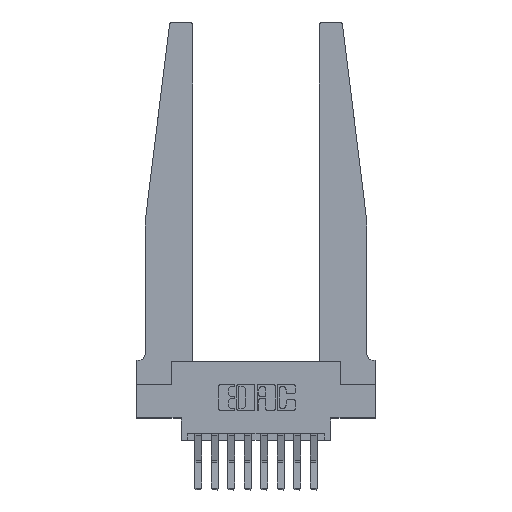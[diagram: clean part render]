
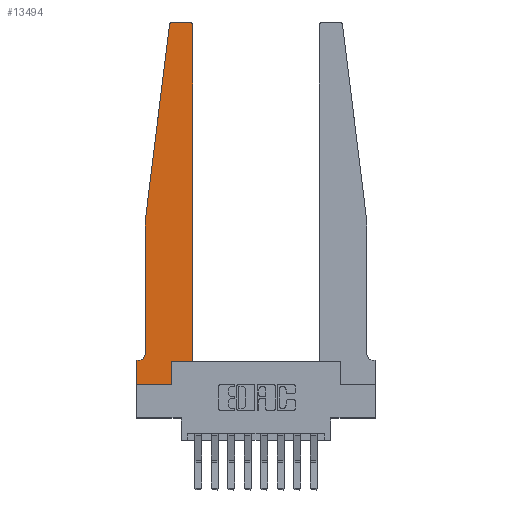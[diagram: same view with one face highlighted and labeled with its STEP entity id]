
A CAD part, top view. The second image highlights one B-rep face of the part: STEP entity #13494.
In plain terms, the highlighted planar face has unit normal (0, 0, 1).
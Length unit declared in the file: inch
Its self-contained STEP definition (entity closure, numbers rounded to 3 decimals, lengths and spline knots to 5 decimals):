
#109 = VECTOR ( 'NONE', #4721, 39.37008 ) ;
#311 = ORIENTED_EDGE ( 'NONE', *, *, #5082, .T. ) ;
#319 = DIRECTION ( 'NONE',  ( 0., 1., 0. ) ) ;
#693 = ORIENTED_EDGE ( 'NONE', *, *, #2034, .T. ) ;
#703 = ORIENTED_EDGE ( 'NONE', *, *, #11220, .T. ) ;
#706 = CARTESIAN_POINT ( 'NONE',  ( 0.27653, 2.72, 0.37 ) ) ;
#908 = AXIS2_PLACEMENT_3D ( 'NONE', #3450, #4506, #8094 ) ;
#1229 = DIRECTION ( 'NONE',  ( 0., -1., 0. ) ) ;
#1250 = EDGE_CURVE ( 'NONE', #2237, #6343, #10101, .T. ) ;
#1474 = LINE ( 'NONE', #10865, #3398 ) ;
#1590 = AXIS2_PLACEMENT_3D ( 'NONE', #5917, #10556, #12864 ) ;
#1916 = VECTOR ( 'NONE', #14478, 39.37008 ) ;
#1954 = VECTOR ( 'NONE', #14543, 39.37008 ) ;
#2034 = EDGE_CURVE ( 'NONE', #4406, #7378, #13529, .T. ) ;
#2237 = VERTEX_POINT ( 'NONE', #14518 ) ;
#2655 = CARTESIAN_POINT ( 'NONE',  ( 0., 0., 0.37 ) ) ;
#2933 = VECTOR ( 'NONE', #10712, 39.37008 ) ;
#3125 = CARTESIAN_POINT ( 'NONE',  ( 0.395, 2.75, 0.37 ) ) ;
#3334 = LINE ( 'NONE', #13623, #9030 ) ;
#3358 = CARTESIAN_POINT ( 'NONE',  ( 0.2605, 0.18, 0.37 ) ) ;
#3398 = VECTOR ( 'NONE', #319, 39.37008 ) ;
#3450 = CARTESIAN_POINT ( 'NONE',  ( 0.395, 2.72, 0.37 ) ) ;
#3584 = EDGE_CURVE ( 'NONE', #11064, #14182, #9532, .T. ) ;
#3735 = EDGE_CURVE ( 'NONE', #7490, #5936, #10942, .T. ) ;
#4406 = VERTEX_POINT ( 'NONE', #9336 ) ;
#4506 = DIRECTION ( 'NONE',  ( 0., 0., 1. ) ) ;
#4616 = VERTEX_POINT ( 'NONE', #4710 ) ;
#4710 = CARTESIAN_POINT ( 'NONE',  ( 0.425, 0.18, 0.37 ) ) ;
#4721 = DIRECTION ( 'NONE',  ( 0., -1., 0. ) ) ;
#5082 = EDGE_CURVE ( 'NONE', #14182, #4406, #9663, .T. ) ;
#5093 = CARTESIAN_POINT ( 'NONE',  ( 0.065, 0.1875, 0.37 ) ) ;
#5604 = DIRECTION ( 'NONE',  ( 0., 1., 0. ) ) ;
#5658 = ORIENTED_EDGE ( 'NONE', *, *, #12893, .T. ) ;
#5861 = CARTESIAN_POINT ( 'NONE',  ( 0.2605, 0., 0.37 ) ) ;
#5902 = CARTESIAN_POINT ( 'NONE',  ( 0., 0.1875, 0.37 ) ) ;
#5917 = CARTESIAN_POINT ( 'NONE',  ( 0.015, 0.2375, 0.37 ) ) ;
#5936 = VERTEX_POINT ( 'NONE', #5902 ) ;
#6343 = VERTEX_POINT ( 'NONE', #5861 ) ;
#6803 = CARTESIAN_POINT ( 'NONE',  ( 0., 0.1875, 0.37 ) ) ;
#6869 = ORIENTED_EDGE ( 'NONE', *, *, #14521, .T. ) ;
#6882 = EDGE_LOOP ( 'NONE', ( #311, #693, #12011, #10905, #12956, #14934, #6869, #10841, #7657, #5658, #703, #12713 ) ) ;
#7037 = CARTESIAN_POINT ( 'NONE',  ( 0.065, 1.25, 0.37 ) ) ;
#7294 = DIRECTION ( 'NONE',  ( 1., 0., 0. ) ) ;
#7378 = VERTEX_POINT ( 'NONE', #14628 ) ;
#7490 = VERTEX_POINT ( 'NONE', #10343 ) ;
#7521 = LINE ( 'NONE', #11082, #12402 ) ;
#7657 = ORIENTED_EDGE ( 'NONE', *, *, #11694, .T. ) ;
#7905 = AXIS2_PLACEMENT_3D ( 'NONE', #6803, #10142, #14659 ) ;
#8094 = DIRECTION ( 'NONE',  ( 1., 0., 0. ) ) ;
#8224 = CIRCLE ( 'NONE', #1590, 0.05 ) ;
#8371 = VERTEX_POINT ( 'NONE', #7037 ) ;
#8424 = VERTEX_POINT ( 'NONE', #9612 ) ;
#8801 = DIRECTION ( 'NONE',  ( 1., 0., 0. ) ) ;
#8982 = PLANE ( 'NONE',  #7905 ) ;
#9030 = VECTOR ( 'NONE', #5604, 39.37008 ) ;
#9336 = CARTESIAN_POINT ( 'NONE',  ( 0.27653, 2.75, 0.37 ) ) ;
#9532 = CIRCLE ( 'NONE', #908, 0.03 ) ;
#9612 = CARTESIAN_POINT ( 'NONE',  ( 0.065, 0.2375, 0.37 ) ) ;
#9663 = LINE ( 'NONE', #14399, #1916 ) ;
#9741 = VERTEX_POINT ( 'NONE', #3358 ) ;
#9867 = CARTESIAN_POINT ( 'NONE',  ( 0., 0., 0.37 ) ) ;
#10101 = LINE ( 'NONE', #9867, #1954 ) ;
#10142 = DIRECTION ( 'NONE',  ( 0., 0., 1. ) ) ;
#10343 = CARTESIAN_POINT ( 'NONE',  ( 0.015, 0.1875, 0.37 ) ) ;
#10527 = DIRECTION ( 'NONE',  ( -0.122, -0.992, 0. ) ) ;
#10556 = DIRECTION ( 'NONE',  ( 0., 0., -1. ) ) ;
#10642 = CARTESIAN_POINT ( 'NONE',  ( 0.425, 2.72, 0.37 ) ) ;
#10712 = DIRECTION ( 'NONE',  ( -1., 0., 0. ) ) ;
#10841 = ORIENTED_EDGE ( 'NONE', *, *, #1250, .T. ) ;
#10865 = CARTESIAN_POINT ( 'NONE',  ( 0.425, 0.18, 0.37 ) ) ;
#10905 = ORIENTED_EDGE ( 'NONE', *, *, #12795, .T. ) ;
#10942 = LINE ( 'NONE', #5093, #2933 ) ;
#11064 = VERTEX_POINT ( 'NONE', #10642 ) ;
#11082 = CARTESIAN_POINT ( 'NONE',  ( 0.425, 0.18, 0.37 ) ) ;
#11216 = FACE_OUTER_BOUND ( 'NONE', #6882, .T. ) ;
#11220 = EDGE_CURVE ( 'NONE', #4616, #11064, #1474, .T. ) ;
#11413 = VECTOR ( 'NONE', #10527, 39.37008 ) ;
#11694 = EDGE_CURVE ( 'NONE', #6343, #9741, #3334, .T. ) ;
#11925 = CARTESIAN_POINT ( 'NONE',  ( 0.065, 1.25, 0.37 ) ) ;
#12011 = ORIENTED_EDGE ( 'NONE', *, *, #14855, .T. ) ;
#12402 = VECTOR ( 'NONE', #7294, 39.37008 ) ;
#12537 = CARTESIAN_POINT ( 'NONE',  ( 0.065, 1.25, 0.37 ) ) ;
#12713 = ORIENTED_EDGE ( 'NONE', *, *, #3584, .T. ) ;
#12779 = EDGE_CURVE ( 'NONE', #8424, #7490, #8224, .T. ) ;
#12795 = EDGE_CURVE ( 'NONE', #8371, #8424, #15218, .T. ) ;
#12864 = DIRECTION ( 'NONE',  ( -1., 0., 0. ) ) ;
#12893 = EDGE_CURVE ( 'NONE', #9741, #4616, #7521, .T. ) ;
#12956 = ORIENTED_EDGE ( 'NONE', *, *, #12779, .T. ) ;
#13171 = LINE ( 'NONE', #2655, #13860 ) ;
#13427 = DIRECTION ( 'NONE',  ( 0., 0., 1. ) ) ;
#13494 = ADVANCED_FACE ( 'NONE', ( #11216 ), #8982, .T. ) ;
#13529 = CIRCLE ( 'NONE', #15210, 0.03 ) ;
#13623 = CARTESIAN_POINT ( 'NONE',  ( 0.2605, 0.18, 0.37 ) ) ;
#13860 = VECTOR ( 'NONE', #1229, 39.37008 ) ;
#14054 = LINE ( 'NONE', #12537, #11413 ) ;
#14182 = VERTEX_POINT ( 'NONE', #3125 ) ;
#14399 = CARTESIAN_POINT ( 'NONE',  ( 0.25, 2.75, 0.37 ) ) ;
#14478 = DIRECTION ( 'NONE',  ( -1., 0., 0. ) ) ;
#14518 = CARTESIAN_POINT ( 'NONE',  ( 0., 0., 0.37 ) ) ;
#14521 = EDGE_CURVE ( 'NONE', #5936, #2237, #13171, .T. ) ;
#14543 = DIRECTION ( 'NONE',  ( 1., 0., 0. ) ) ;
#14628 = CARTESIAN_POINT ( 'NONE',  ( 0.24675, 2.72367, 0.37 ) ) ;
#14659 = DIRECTION ( 'NONE',  ( 1., 0., 0. ) ) ;
#14855 = EDGE_CURVE ( 'NONE', #7378, #8371, #14054, .T. ) ;
#14934 = ORIENTED_EDGE ( 'NONE', *, *, #3735, .T. ) ;
#15210 = AXIS2_PLACEMENT_3D ( 'NONE', #706, #13427, #8801 ) ;
#15218 = LINE ( 'NONE', #11925, #109 ) ;
